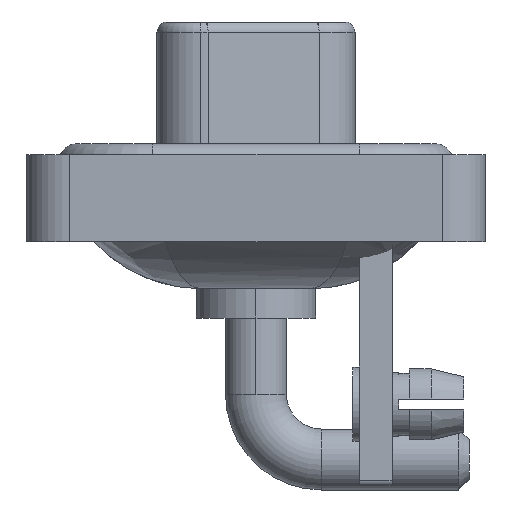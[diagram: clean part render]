
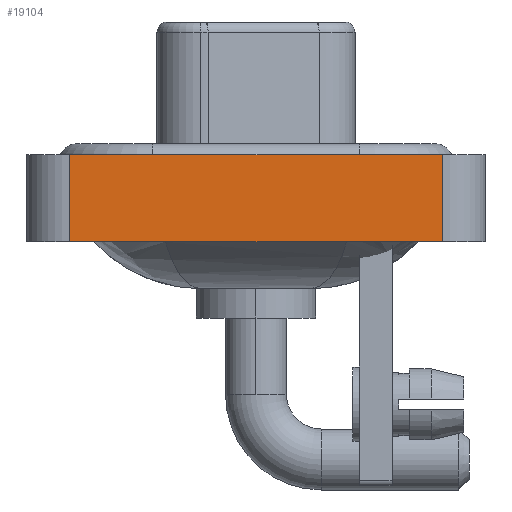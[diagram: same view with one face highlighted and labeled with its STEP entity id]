
A CAD part, left-side view. The second image highlights one B-rep face of the part: STEP entity #19104.
In plain terms, the highlighted planar face has unit normal (-1, 0, 0).
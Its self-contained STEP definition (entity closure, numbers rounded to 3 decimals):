
#68 = ORIENTED_EDGE ( 'NONE', *, *, #719, .F. ) ;
#195 = LINE ( 'NONE', #12858, #10697 ) ;
#719 = EDGE_CURVE ( 'NONE', #14513, #13043, #20199, .T. ) ;
#2375 = LINE ( 'NONE', #3637, #3703 ) ;
#2990 = PLANE ( 'NONE',  #6023 ) ;
#3222 = CARTESIAN_POINT ( 'NONE',  ( -7.35, 8.55, 0.4 ) ) ;
#3637 = CARTESIAN_POINT ( 'NONE',  ( -7.35, 8.55, -3.6 ) ) ;
#3703 = VECTOR ( 'NONE', #9347, 1000. ) ;
#4318 = EDGE_LOOP ( 'NONE', ( #17033, #68, #13761, #14225 ) ) ;
#4692 = DIRECTION ( 'NONE',  ( 0., -1., 0. ) ) ;
#5293 = VECTOR ( 'NONE', #17009, 1000. ) ;
#6023 = AXIS2_PLACEMENT_3D ( 'NONE', #10665, #9449, #7464 ) ;
#6120 = FACE_OUTER_BOUND ( 'NONE', #4318, .T. ) ;
#6339 = VECTOR ( 'NONE', #11381, 1000. ) ;
#7464 = DIRECTION ( 'NONE',  ( 0., 0., 1. ) ) ;
#9262 = VERTEX_POINT ( 'NONE', #16379 ) ;
#9341 = EDGE_CURVE ( 'NONE', #13525, #14513, #2375, .T. ) ;
#9347 = DIRECTION ( 'NONE',  ( 0., 0., 1. ) ) ;
#9449 = DIRECTION ( 'NONE',  ( -1., 0., 0. ) ) ;
#10665 = CARTESIAN_POINT ( 'NONE',  ( -7.35, -8.55, -3.6 ) ) ;
#10697 = VECTOR ( 'NONE', #4692, 1000. ) ;
#11213 = EDGE_CURVE ( 'NONE', #9262, #13043, #11276, .T. ) ;
#11251 = CARTESIAN_POINT ( 'NONE',  ( -7.35, 8.55, -3.6 ) ) ;
#11276 = LINE ( 'NONE', #12731, #6339 ) ;
#11381 = DIRECTION ( 'NONE',  ( 0., 0., 1. ) ) ;
#12450 = CARTESIAN_POINT ( 'NONE',  ( -7.35, -8.55, 0.4 ) ) ;
#12731 = CARTESIAN_POINT ( 'NONE',  ( -7.35, -8.55, -3.6 ) ) ;
#12858 = CARTESIAN_POINT ( 'NONE',  ( -7.35, -8.55, -3.6 ) ) ;
#13043 = VERTEX_POINT ( 'NONE', #17376 ) ;
#13525 = VERTEX_POINT ( 'NONE', #11251 ) ;
#13761 = ORIENTED_EDGE ( 'NONE', *, *, #9341, .F. ) ;
#14225 = ORIENTED_EDGE ( 'NONE', *, *, #17613, .T. ) ;
#14513 = VERTEX_POINT ( 'NONE', #3222 ) ;
#16379 = CARTESIAN_POINT ( 'NONE',  ( -7.35, -8.55, -3.6 ) ) ;
#17009 = DIRECTION ( 'NONE',  ( 0., -1., 0. ) ) ;
#17033 = ORIENTED_EDGE ( 'NONE', *, *, #11213, .T. ) ;
#17376 = CARTESIAN_POINT ( 'NONE',  ( -7.35, -8.55, 0.4 ) ) ;
#17613 = EDGE_CURVE ( 'NONE', #13525, #9262, #195, .T. ) ;
#19104 = ADVANCED_FACE ( 'NONE', ( #6120 ), #2990, .T. ) ;
#20199 = LINE ( 'NONE', #12450, #5293 ) ;
